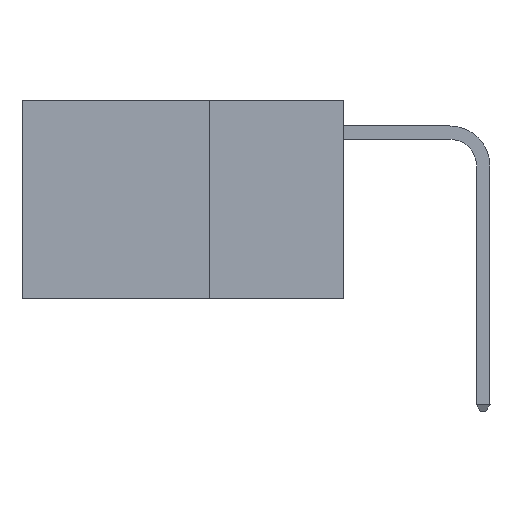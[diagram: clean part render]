
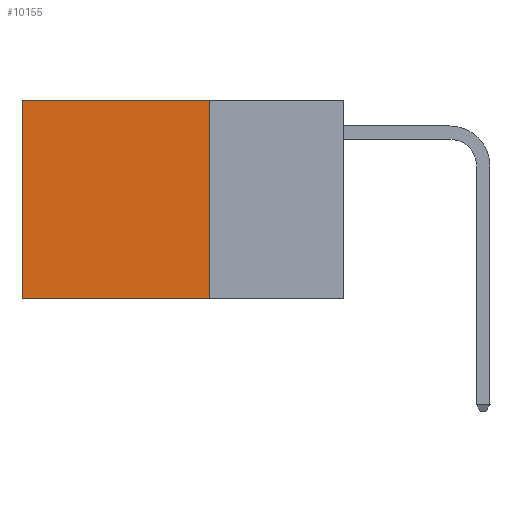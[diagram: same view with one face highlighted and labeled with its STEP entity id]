
A CAD part, left-side view. The second image highlights one B-rep face of the part: STEP entity #10155.
In plain terms, the highlighted planar face has unit normal (-1, 0, 0).
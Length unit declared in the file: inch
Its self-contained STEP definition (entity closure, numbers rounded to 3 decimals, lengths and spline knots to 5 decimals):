
#326 = CARTESIAN_POINT ( 'NONE',  ( 0.2625, 0.25, 0. ) ) ;
#2453 = EDGE_CURVE ( 'NONE', #17190, #16661, #13184, .T. ) ;
#3260 = VERTEX_POINT ( 'NONE', #17522 ) ;
#3661 = ORIENTED_EDGE ( 'NONE', *, *, #2453, .F. ) ;
#4267 = EDGE_CURVE ( 'NONE', #3260, #14906, #10605, .T. ) ;
#5475 = LINE ( 'NONE', #14409, #22195 ) ;
#6320 = CARTESIAN_POINT ( 'NONE',  ( 0.2625, 0.25, -0.37 ) ) ;
#6766 = LINE ( 'NONE', #326, #14427 ) ;
#7339 = FACE_OUTER_BOUND ( 'NONE', #27781, .T. ) ;
#8136 = CARTESIAN_POINT ( 'NONE',  ( 0.2625, 0.6, 0. ) ) ;
#8856 = VECTOR ( 'NONE', #10676, 39.37008 ) ;
#9554 = DIRECTION ( 'NONE',  ( 0., 0., -1. ) ) ;
#9703 = DIRECTION ( 'NONE',  ( 1., 0., 0. ) ) ;
#9786 = CARTESIAN_POINT ( 'NONE',  ( 0.2625, 0.6, -0.37 ) ) ;
#10046 = EDGE_CURVE ( 'NONE', #3260, #17190, #6766, .T. ) ;
#10155 = ADVANCED_FACE ( 'NONE', ( #7339 ), #25259, .F. ) ;
#10393 = CARTESIAN_POINT ( 'NONE',  ( 0.2625, 0.25, -0.37 ) ) ;
#10605 = LINE ( 'NONE', #19566, #19217 ) ;
#10676 = DIRECTION ( 'NONE',  ( 0., 1., 0. ) ) ;
#11113 = ORIENTED_EDGE ( 'NONE', *, *, #4267, .T. ) ;
#11946 = DIRECTION ( 'NONE',  ( 0., 0., -1. ) ) ;
#13184 = LINE ( 'NONE', #10393, #8856 ) ;
#14409 = CARTESIAN_POINT ( 'NONE',  ( 0.2625, 0.6, 0. ) ) ;
#14427 = VECTOR ( 'NONE', #18247, 39.37008 ) ;
#14906 = VERTEX_POINT ( 'NONE', #8136 ) ;
#16661 = VERTEX_POINT ( 'NONE', #9786 ) ;
#16729 = ORIENTED_EDGE ( 'NONE', *, *, #28667, .T. ) ;
#17190 = VERTEX_POINT ( 'NONE', #6320 ) ;
#17522 = CARTESIAN_POINT ( 'NONE',  ( 0.2625, 0.25, 0. ) ) ;
#18247 = DIRECTION ( 'NONE',  ( 0., 0., -1. ) ) ;
#18714 = AXIS2_PLACEMENT_3D ( 'NONE', #23218, #9703, #9554 ) ;
#19146 = DIRECTION ( 'NONE',  ( 0., 1., 0. ) ) ;
#19217 = VECTOR ( 'NONE', #19146, 39.37008 ) ;
#19566 = CARTESIAN_POINT ( 'NONE',  ( 0.2625, 0.25, 0. ) ) ;
#22195 = VECTOR ( 'NONE', #11946, 39.37008 ) ;
#23218 = CARTESIAN_POINT ( 'NONE',  ( 0.2625, 0.25, 0. ) ) ;
#24039 = ORIENTED_EDGE ( 'NONE', *, *, #10046, .F. ) ;
#25259 = PLANE ( 'NONE',  #18714 ) ;
#27781 = EDGE_LOOP ( 'NONE', ( #16729, #3661, #24039, #11113 ) ) ;
#28667 = EDGE_CURVE ( 'NONE', #14906, #16661, #5475, .T. ) ;
